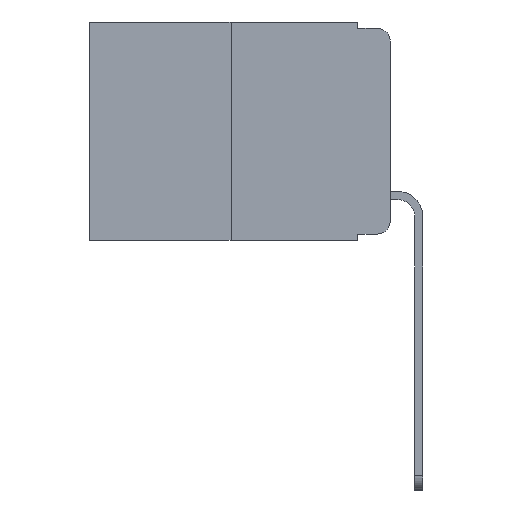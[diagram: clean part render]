
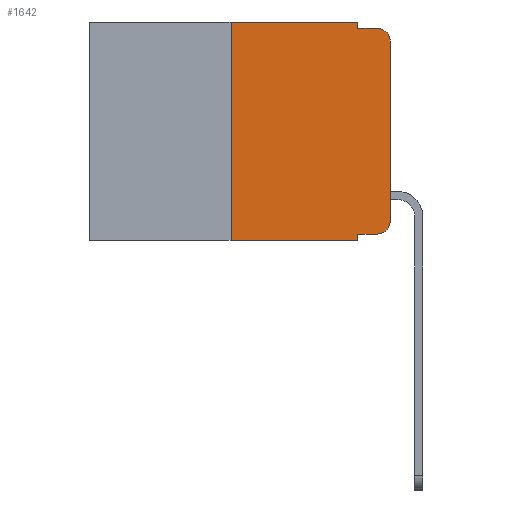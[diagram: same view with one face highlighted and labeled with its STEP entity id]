
A CAD part, left-side view. The second image highlights one B-rep face of the part: STEP entity #1642.
In plain terms, the highlighted planar face has unit normal (-1, 0, 0).
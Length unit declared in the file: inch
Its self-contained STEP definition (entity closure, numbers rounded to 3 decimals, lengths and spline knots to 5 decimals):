
#28 = EDGE_CURVE ( 'NONE', #7005, #6671, #4917, .T. ) ;
#105 = ORIENTED_EDGE ( 'NONE', *, *, #6530, .F. ) ;
#207 = DIRECTION ( 'NONE',  ( -1., 0., 0. ) ) ;
#386 = CIRCLE ( 'NONE', #9762, 0.02 ) ;
#492 = CARTESIAN_POINT ( 'NONE',  ( 0., 0.051, -0.01 ) ) ;
#695 = ORIENTED_EDGE ( 'NONE', *, *, #1447, .T. ) ;
#1360 = DIRECTION ( 'NONE',  ( 0., 0., 1. ) ) ;
#1447 = EDGE_CURVE ( 'NONE', #7388, #13009, #10687, .T. ) ;
#1569 = CARTESIAN_POINT ( 'NONE',  ( 0., 0.051, -0.333 ) ) ;
#1642 = ADVANCED_FACE ( 'NONE', ( #2508 ), #7975, .F. ) ;
#2440 = ORIENTED_EDGE ( 'NONE', *, *, #13455, .F. ) ;
#2478 = EDGE_CURVE ( 'NONE', #13009, #9609, #11789, .T. ) ;
#2508 = FACE_OUTER_BOUND ( 'NONE', #6967, .T. ) ;
#2606 = EDGE_CURVE ( 'NONE', #3764, #7745, #4591, .T. ) ;
#2633 = CARTESIAN_POINT ( 'NONE',  ( 0., 0.051, 0. ) ) ;
#2713 = CARTESIAN_POINT ( 'NONE',  ( 0., 0.473, -0.343 ) ) ;
#2777 = DIRECTION ( 'NONE',  ( 1., 0., 0. ) ) ;
#3055 = CARTESIAN_POINT ( 'NONE',  ( 0., 0.473, 0. ) ) ;
#3298 = VECTOR ( 'NONE', #11620, 39.37008 ) ;
#3764 = VERTEX_POINT ( 'NONE', #11493 ) ;
#3966 = DIRECTION ( 'NONE',  ( 0., 0., 1. ) ) ;
#4045 = CARTESIAN_POINT ( 'NONE',  ( 0., 0., -0.313 ) ) ;
#4087 = ORIENTED_EDGE ( 'NONE', *, *, #11573, .T. ) ;
#4297 = CARTESIAN_POINT ( 'NONE',  ( 0., 0.051, -0.343 ) ) ;
#4579 = VECTOR ( 'NONE', #13000, 39.37008 ) ;
#4585 = AXIS2_PLACEMENT_3D ( 'NONE', #11097, #2777, #10077 ) ;
#4591 = LINE ( 'NONE', #6299, #7035 ) ;
#4606 = VECTOR ( 'NONE', #6153, 39.37008 ) ;
#4659 = ORIENTED_EDGE ( 'NONE', *, *, #28, .F. ) ;
#4701 = ORIENTED_EDGE ( 'NONE', *, *, #2606, .F. ) ;
#4801 = CARTESIAN_POINT ( 'NONE',  ( 0., 0.02, -0.333 ) ) ;
#4917 = LINE ( 'NONE', #3055, #4606 ) ;
#4960 = VECTOR ( 'NONE', #1360, 39.37008 ) ;
#5218 = CARTESIAN_POINT ( 'NONE',  ( 0., 0.25, 0. ) ) ;
#5258 = DIRECTION ( 'NONE',  ( 0., 0., -1. ) ) ;
#5301 = LINE ( 'NONE', #9729, #4960 ) ;
#5443 = DIRECTION ( 'NONE',  ( -1., 0., 0. ) ) ;
#6153 = DIRECTION ( 'NONE',  ( 0., -1., 0. ) ) ;
#6299 = CARTESIAN_POINT ( 'NONE',  ( 0., 0.051, 0. ) ) ;
#6351 = CARTESIAN_POINT ( 'NONE',  ( 0., 0., -0.03 ) ) ;
#6477 = CARTESIAN_POINT ( 'NONE',  ( 0., 0.02, -0.03 ) ) ;
#6530 = EDGE_CURVE ( 'NONE', #6671, #7251, #11632, .T. ) ;
#6671 = VERTEX_POINT ( 'NONE', #2633 ) ;
#6967 = EDGE_LOOP ( 'NONE', ( #8573, #11030, #12660, #105, #4659, #2440, #10467, #4701, #4087, #695 ) ) ;
#7005 = VERTEX_POINT ( 'NONE', #5218 ) ;
#7035 = VECTOR ( 'NONE', #5258, 39.37008 ) ;
#7251 = VERTEX_POINT ( 'NONE', #12915 ) ;
#7312 = EDGE_CURVE ( 'NONE', #7251, #9726, #8013, .T. ) ;
#7388 = VERTEX_POINT ( 'NONE', #4801 ) ;
#7540 = DIRECTION ( 'NONE',  ( 0., 0., -1. ) ) ;
#7745 = VERTEX_POINT ( 'NONE', #4297 ) ;
#7799 = VECTOR ( 'NONE', #7837, 39.37008 ) ;
#7837 = DIRECTION ( 'NONE',  ( 0., -1., 0. ) ) ;
#7975 = PLANE ( 'NONE',  #4585 ) ;
#8013 = LINE ( 'NONE', #492, #4579 ) ;
#8350 = AXIS2_PLACEMENT_3D ( 'NONE', #11698, #5443, #12736 ) ;
#8573 = ORIENTED_EDGE ( 'NONE', *, *, #2478, .T. ) ;
#8595 = CARTESIAN_POINT ( 'NONE',  ( 0., 0.02, -0.01 ) ) ;
#9580 = LINE ( 'NONE', #2713, #12332 ) ;
#9609 = VERTEX_POINT ( 'NONE', #6351 ) ;
#9726 = VERTEX_POINT ( 'NONE', #8595 ) ;
#9729 = CARTESIAN_POINT ( 'NONE',  ( 0., 0.25, 0. ) ) ;
#9762 = AXIS2_PLACEMENT_3D ( 'NONE', #6477, #207, #7540 ) ;
#10019 = DIRECTION ( 'NONE',  ( 0., -1., 0. ) ) ;
#10077 = DIRECTION ( 'NONE',  ( 0., 0., -1. ) ) ;
#10467 = ORIENTED_EDGE ( 'NONE', *, *, #12162, .T. ) ;
#10576 = CARTESIAN_POINT ( 'NONE',  ( 0., 0.051, 0. ) ) ;
#10687 = CIRCLE ( 'NONE', #8350, 0.02 ) ;
#10914 = LINE ( 'NONE', #1569, #7799 ) ;
#11030 = ORIENTED_EDGE ( 'NONE', *, *, #13376, .T. ) ;
#11097 = CARTESIAN_POINT ( 'NONE',  ( 0., 0.473, 0. ) ) ;
#11467 = VECTOR ( 'NONE', #3966, 39.37008 ) ;
#11471 = VERTEX_POINT ( 'NONE', #12842 ) ;
#11493 = CARTESIAN_POINT ( 'NONE',  ( 0., 0.051, -0.333 ) ) ;
#11573 = EDGE_CURVE ( 'NONE', #3764, #7388, #10914, .T. ) ;
#11620 = DIRECTION ( 'NONE',  ( 0., 0., -1. ) ) ;
#11632 = LINE ( 'NONE', #10576, #3298 ) ;
#11698 = CARTESIAN_POINT ( 'NONE',  ( 0., 0.02, -0.313 ) ) ;
#11789 = LINE ( 'NONE', #13349, #11467 ) ;
#12162 = EDGE_CURVE ( 'NONE', #11471, #7745, #9580, .T. ) ;
#12332 = VECTOR ( 'NONE', #10019, 39.37008 ) ;
#12660 = ORIENTED_EDGE ( 'NONE', *, *, #7312, .F. ) ;
#12736 = DIRECTION ( 'NONE',  ( 0., 0., -1. ) ) ;
#12842 = CARTESIAN_POINT ( 'NONE',  ( 0., 0.25, -0.343 ) ) ;
#12915 = CARTESIAN_POINT ( 'NONE',  ( 0., 0.051, -0.01 ) ) ;
#13000 = DIRECTION ( 'NONE',  ( 0., -1., 0. ) ) ;
#13009 = VERTEX_POINT ( 'NONE', #4045 ) ;
#13349 = CARTESIAN_POINT ( 'NONE',  ( 0., 0., 0. ) ) ;
#13376 = EDGE_CURVE ( 'NONE', #9609, #9726, #386, .T. ) ;
#13455 = EDGE_CURVE ( 'NONE', #11471, #7005, #5301, .T. ) ;
